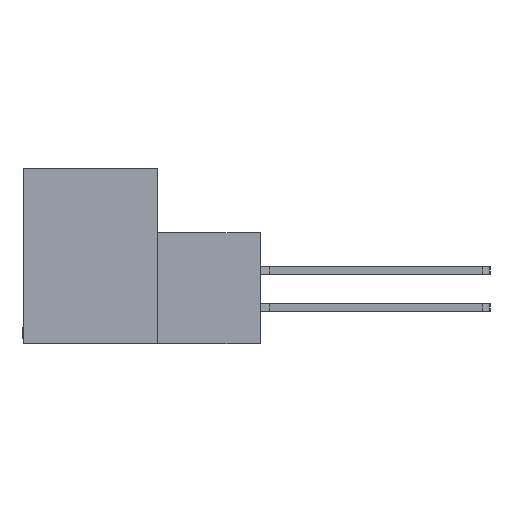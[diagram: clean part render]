
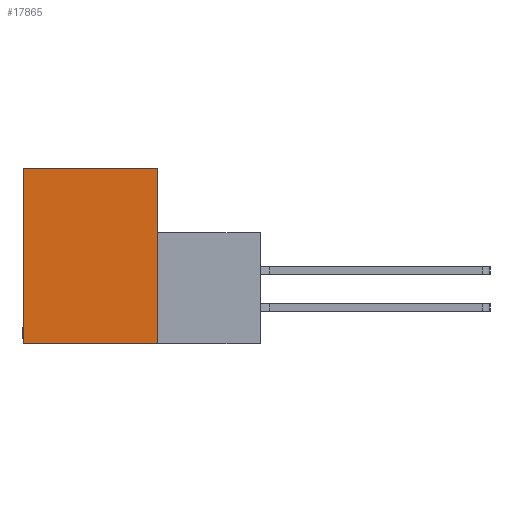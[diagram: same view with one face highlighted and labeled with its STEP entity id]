
A CAD part, left-side view. The second image highlights one B-rep face of the part: STEP entity #17865.
In plain terms, the highlighted planar face has unit normal (-1, 0, 0).
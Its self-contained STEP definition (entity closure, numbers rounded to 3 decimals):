
#2772 = VECTOR ( 'NONE', #17925, 1000. ) ;
#4928 = VECTOR ( 'NONE', #35838, 1000. ) ;
#5391 = EDGE_CURVE ( 'NONE', #27761, #26242, #33997, .T. ) ;
#7354 = ORIENTED_EDGE ( 'NONE', *, *, #5391, .F. ) ;
#9871 = CARTESIAN_POINT ( 'NONE',  ( 0., 11.506, -15.088 ) ) ;
#10497 = VECTOR ( 'NONE', #15085, 1000. ) ;
#10661 = CARTESIAN_POINT ( 'NONE',  ( 0., 0., 0. ) ) ;
#11220 = FACE_OUTER_BOUND ( 'NONE', #50208, .T. ) ;
#11343 = EDGE_CURVE ( 'NONE', #26242, #31245, #27844, .T. ) ;
#12226 = CARTESIAN_POINT ( 'NONE',  ( 0., 11.506, 0. ) ) ;
#12417 = CARTESIAN_POINT ( 'NONE',  ( 0., 0., 0. ) ) ;
#15016 = DIRECTION ( 'NONE',  ( 0., 0., -1. ) ) ;
#15085 = DIRECTION ( 'NONE',  ( 0., 1., 0. ) ) ;
#16472 = CARTESIAN_POINT ( 'NONE',  ( 0., 0., 0. ) ) ;
#17793 = AXIS2_PLACEMENT_3D ( 'NONE', #10661, #30750, #15016 ) ;
#17865 = ADVANCED_FACE ( 'NONE', ( #11220 ), #34378, .F. ) ;
#17925 = DIRECTION ( 'NONE',  ( 0., -1., 0. ) ) ;
#19467 = LINE ( 'NONE', #43019, #20705 ) ;
#20705 = VECTOR ( 'NONE', #35257, 1000. ) ;
#25290 = ORIENTED_EDGE ( 'NONE', *, *, #48459, .F. ) ;
#26242 = VERTEX_POINT ( 'NONE', #41097 ) ;
#27761 = VERTEX_POINT ( 'NONE', #12417 ) ;
#27844 = LINE ( 'NONE', #51185, #10497 ) ;
#28682 = ORIENTED_EDGE ( 'NONE', *, *, #50329, .F. ) ;
#29262 = CARTESIAN_POINT ( 'NONE',  ( 0., 11.506, 0. ) ) ;
#30750 = DIRECTION ( 'NONE',  ( 1., 0., 0. ) ) ;
#31245 = VERTEX_POINT ( 'NONE', #9871 ) ;
#31263 = VERTEX_POINT ( 'NONE', #29262 ) ;
#33997 = LINE ( 'NONE', #16472, #4928 ) ;
#34378 = PLANE ( 'NONE',  #17793 ) ;
#35004 = ORIENTED_EDGE ( 'NONE', *, *, #11343, .F. ) ;
#35257 = DIRECTION ( 'NONE',  ( 0., 0., 1. ) ) ;
#35838 = DIRECTION ( 'NONE',  ( 0., 0., -1. ) ) ;
#38658 = LINE ( 'NONE', #12226, #2772 ) ;
#41097 = CARTESIAN_POINT ( 'NONE',  ( 0., 0., -15.088 ) ) ;
#43019 = CARTESIAN_POINT ( 'NONE',  ( 0., 11.506, -15.088 ) ) ;
#48459 = EDGE_CURVE ( 'NONE', #31245, #31263, #19467, .T. ) ;
#50208 = EDGE_LOOP ( 'NONE', ( #35004, #7354, #28682, #25290 ) ) ;
#50329 = EDGE_CURVE ( 'NONE', #31263, #27761, #38658, .T. ) ;
#51185 = CARTESIAN_POINT ( 'NONE',  ( 0., -8.814, -15.088 ) ) ;
